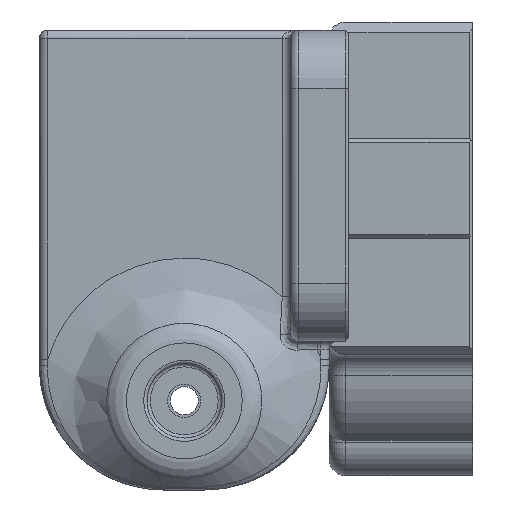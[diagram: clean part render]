
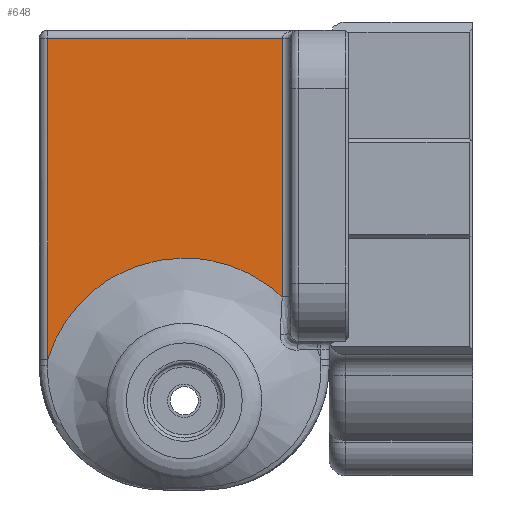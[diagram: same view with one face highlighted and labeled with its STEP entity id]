
A CAD part, front view. The second image highlights one B-rep face of the part: STEP entity #648.
In plain terms, the highlighted planar face has unit normal (0, -1, 0).
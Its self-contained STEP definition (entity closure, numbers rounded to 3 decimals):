
#403 = LINE ( 'NONE', #5251, #7152 ) ;
#423 = VECTOR ( 'NONE', #5421, 1000. ) ;
#497 = ORIENTED_EDGE ( 'NONE', *, *, #1219, .F. ) ;
#538 = VERTEX_POINT ( 'NONE', #5384 ) ;
#584 = VECTOR ( 'NONE', #2071, 1000. ) ;
#648 = ADVANCED_FACE ( 'NONE', ( #8157 ), #5777, .F. ) ;
#810 = CARTESIAN_POINT ( 'NONE',  ( -213.516, -0.918, 19.1 ) ) ;
#970 = B_SPLINE_CURVE_WITH_KNOTS ( 'NONE', 3,
 ( #3878, #5893, #7871, #6599, #7356, #1326 ),
 .UNSPECIFIED., .F., .F.,
 ( 4, 1, 1, 4 ),
 ( -1.112, -0.768, -0.383, 0.001 ),
 .UNSPECIFIED. ) ;
#1142 = VERTEX_POINT ( 'NONE', #1228 ) ;
#1178 = B_SPLINE_CURVE_WITH_KNOTS ( 'NONE', 3,
 ( #2947, #5650, #4477, #6476, #2546, #8424, #1833 ),
 .UNSPECIFIED., .F., .F.,
 ( 4, 1, 2, 4 ),
 ( 1.115, 1.156, 1.54, 2.189 ),
 .UNSPECIFIED. ) ;
#1219 = EDGE_CURVE ( 'NONE', #3625, #1142, #3365, .T. ) ;
#1228 = CARTESIAN_POINT ( 'NONE',  ( -203.098, -0.918, -10.924 ) ) ;
#1326 = CARTESIAN_POINT ( 'NONE',  ( -213.533, -0.918, -7.42 ) ) ;
#1821 = CARTESIAN_POINT ( 'NONE',  ( -201.682, -0.918, 19.1 ) ) ;
#1833 = CARTESIAN_POINT ( 'NONE',  ( -230.014, -0.918, -19.646 ) ) ;
#1904 = CARTESIAN_POINT ( 'NONE',  ( -201.682, -0.918, 8.994 ) ) ;
#1972 = DIRECTION ( 'NONE',  ( 0., 0., 1. ) ) ;
#2014 = CARTESIAN_POINT ( 'NONE',  ( -201.682, -0.918, -12.122 ) ) ;
#2048 = EDGE_CURVE ( 'NONE', #1142, #538, #970, .T. ) ;
#2071 = DIRECTION ( 'NONE',  ( 0., 0., -1. ) ) ;
#2073 = CARTESIAN_POINT ( 'NONE',  ( -202.605, -0.918, -11.298 ) ) ;
#2480 = ORIENTED_EDGE ( 'NONE', *, *, #2632, .F. ) ;
#2526 = ORIENTED_EDGE ( 'NONE', *, *, #7748, .F. ) ;
#2546 = CARTESIAN_POINT ( 'NONE',  ( -228.349, -0.918, -15.606 ) ) ;
#2622 = EDGE_CURVE ( 'NONE', #2882, #6288, #1178, .T. ) ;
#2632 = EDGE_CURVE ( 'NONE', #538, #2882, #2677, .T. ) ;
#2677 = B_SPLINE_CURVE_WITH_KNOTS ( 'NONE', 3,
 ( #3160, #5173, #3141, #7042, #4393, #8347 ),
 .UNSPECIFIED., .F., .F.,
 ( 4, 2, 4 ),
 ( 0.002, 0.771, 1.115 ),
 .UNSPECIFIED. ) ;
#2882 = VERTEX_POINT ( 'NONE', #4143 ) ;
#2947 = CARTESIAN_POINT ( 'NONE',  ( -223.933, -0.918, -10.924 ) ) ;
#3134 = AXIS2_PLACEMENT_3D ( 'NONE', #7671, #8334, #4488 ) ;
#3141 = CARTESIAN_POINT ( 'NONE',  ( -218.658, -0.918, -8.005 ) ) ;
#3160 = CARTESIAN_POINT ( 'NONE',  ( -213.533, -0.918, -7.42 ) ) ;
#3365 = B_SPLINE_CURVE_WITH_KNOTS ( 'NONE', 3,
 ( #5382, #6561, #2073, #6646 ),
 .UNSPECIFIED., .F., .F.,
 ( 4, 4 ),
 ( -1.296, -1.112 ),
 .UNSPECIFIED. ) ;
#3625 = VERTEX_POINT ( 'NONE', #2014 ) ;
#3817 = VERTEX_POINT ( 'NONE', #8366 ) ;
#3878 = CARTESIAN_POINT ( 'NONE',  ( -203.098, -0.918, -10.924 ) ) ;
#3880 = LINE ( 'NONE', #810, #423 ) ;
#4143 = CARTESIAN_POINT ( 'NONE',  ( -223.933, -0.918, -10.924 ) ) ;
#4378 = VERTEX_POINT ( 'NONE', #1821 ) ;
#4393 = CARTESIAN_POINT ( 'NONE',  ( -223.011, -0.918, -10.226 ) ) ;
#4477 = CARTESIAN_POINT ( 'NONE',  ( -225.172, -0.918, -11.883 ) ) ;
#4488 = DIRECTION ( 'NONE',  ( -1., 0., 0. ) ) ;
#4581 = EDGE_CURVE ( 'NONE', #3817, #4378, #3880, .T. ) ;
#4761 = ORIENTED_EDGE ( 'NONE', *, *, #4581, .F. ) ;
#5173 = CARTESIAN_POINT ( 'NONE',  ( -216.108, -0.918, -7.422 ) ) ;
#5251 = CARTESIAN_POINT ( 'NONE',  ( -230.016, -0.918, -5.442 ) ) ;
#5382 = CARTESIAN_POINT ( 'NONE',  ( -201.682, -0.918, -12.122 ) ) ;
#5384 = CARTESIAN_POINT ( 'NONE',  ( -213.533, -0.918, -7.42 ) ) ;
#5421 = DIRECTION ( 'NONE',  ( 1., 0., 0. ) ) ;
#5650 = CARTESIAN_POINT ( 'NONE',  ( -224.042, -0.918, -11.007 ) ) ;
#5705 = CARTESIAN_POINT ( 'NONE',  ( -230.014, -0.918, -19.646 ) ) ;
#5777 = PLANE ( 'NONE',  #3134 ) ;
#5893 = CARTESIAN_POINT ( 'NONE',  ( -204.019, -0.918, -10.226 ) ) ;
#6041 = LINE ( 'NONE', #1904, #584 ) ;
#6288 = VERTEX_POINT ( 'NONE', #5705 ) ;
#6468 = EDGE_CURVE ( 'NONE', #6288, #3817, #403, .T. ) ;
#6476 = CARTESIAN_POINT ( 'NONE',  ( -226.188, -0.918, -12.897 ) ) ;
#6561 = CARTESIAN_POINT ( 'NONE',  ( -202.132, -0.918, -11.698 ) ) ;
#6599 = CARTESIAN_POINT ( 'NONE',  ( -209.663, -0.918, -7.708 ) ) ;
#6616 = ORIENTED_EDGE ( 'NONE', *, *, #6468, .F. ) ;
#6646 = CARTESIAN_POINT ( 'NONE',  ( -203.098, -0.918, -10.924 ) ) ;
#6835 = ORIENTED_EDGE ( 'NONE', *, *, #2622, .F. ) ;
#6941 = ORIENTED_EDGE ( 'NONE', *, *, #2048, .F. ) ;
#7042 = CARTESIAN_POINT ( 'NONE',  ( -222.019, -0.918, -9.62 ) ) ;
#7152 = VECTOR ( 'NONE', #1972, 1000. ) ;
#7356 = CARTESIAN_POINT ( 'NONE',  ( -212.247, -0.918, -7.419 ) ) ;
#7671 = CARTESIAN_POINT ( 'NONE',  ( -213.516, -0.918, -5.442 ) ) ;
#7748 = EDGE_CURVE ( 'NONE', #4378, #3625, #6041, .T. ) ;
#7821 = EDGE_LOOP ( 'NONE', ( #2526, #4761, #6616, #6835, #2480, #6941, #497 ) ) ;
#7871 = CARTESIAN_POINT ( 'NONE',  ( -206.115, -0.918, -8.942 ) ) ;
#8157 = FACE_OUTER_BOUND ( 'NONE', #7821, .T. ) ;
#8334 = DIRECTION ( 'NONE',  ( 0., 1., 0. ) ) ;
#8347 = CARTESIAN_POINT ( 'NONE',  ( -223.933, -0.918, -10.924 ) ) ;
#8366 = CARTESIAN_POINT ( 'NONE',  ( -230.016, -0.918, 19.1 ) ) ;
#8424 = CARTESIAN_POINT ( 'NONE',  ( -229.378, -0.918, -17.565 ) ) ;
